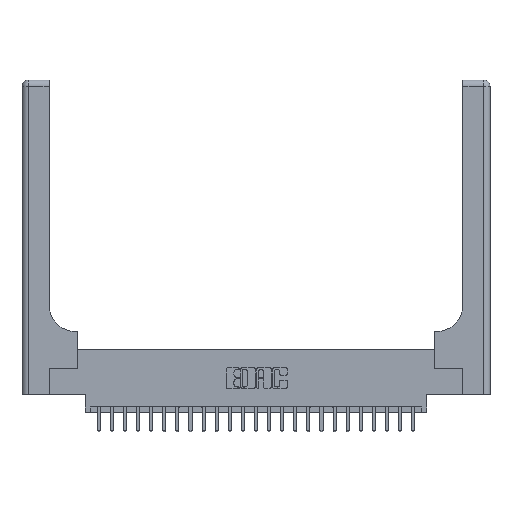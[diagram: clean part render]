
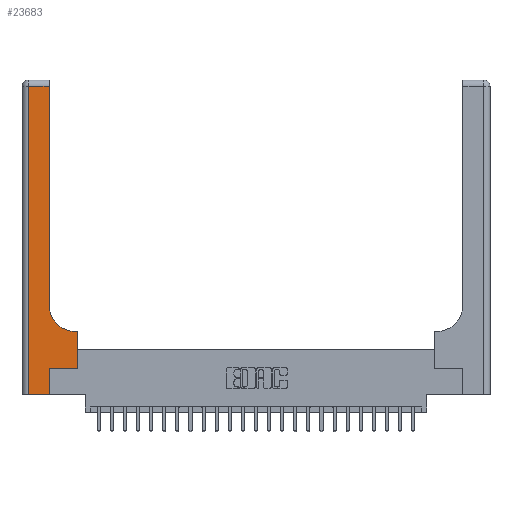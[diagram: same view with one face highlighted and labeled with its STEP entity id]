
A CAD part, top view. The second image highlights one B-rep face of the part: STEP entity #23683.
In plain terms, the highlighted planar face has unit normal (0, 0, 1).
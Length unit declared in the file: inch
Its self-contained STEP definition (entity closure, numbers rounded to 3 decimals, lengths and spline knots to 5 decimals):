
#75 = LINE ( 'NONE', #4916, #19476 ) ;
#496 = VECTOR ( 'NONE', #17481, 39.37008 ) ;
#498 = VERTEX_POINT ( 'NONE', #15207 ) ;
#899 = VECTOR ( 'NONE', #15402, 39.37008 ) ;
#1504 = EDGE_CURVE ( 'NONE', #498, #10730, #18306, .T. ) ;
#1508 = LINE ( 'NONE', #15621, #899 ) ;
#1638 = EDGE_CURVE ( 'NONE', #2886, #498, #1508, .T. ) ;
#1781 = CARTESIAN_POINT ( 'NONE',  ( 0., 0., 0.37 ) ) ;
#1976 = EDGE_CURVE ( 'NONE', #14394, #15338, #6405, .T. ) ;
#2412 = ORIENTED_EDGE ( 'NONE', *, *, #1504, .T. ) ;
#2886 = VERTEX_POINT ( 'NONE', #19608 ) ;
#3238 = CIRCLE ( 'NONE', #21784, 0.25 ) ;
#3376 = VECTOR ( 'NONE', #17264, 39.37008 ) ;
#3769 = DIRECTION ( 'NONE',  ( 1., 0., 0. ) ) ;
#4017 = VECTOR ( 'NONE', #19359, 39.37008 ) ;
#4761 = EDGE_CURVE ( 'NONE', #8968, #14394, #22690, .T. ) ;
#4916 = CARTESIAN_POINT ( 'NONE',  ( 0.528, 0.25, 0.37 ) ) ;
#4970 = DIRECTION ( 'NONE',  ( -1., 0., 0. ) ) ;
#5812 = VERTEX_POINT ( 'NONE', #20276 ) ;
#6086 = FACE_OUTER_BOUND ( 'NONE', #12149, .T. ) ;
#6405 = LINE ( 'NONE', #12341, #14629 ) ;
#6441 = ORIENTED_EDGE ( 'NONE', *, *, #17132, .T. ) ;
#6444 = CARTESIAN_POINT ( 'NONE',  ( 0.06, 3., 0.37 ) ) ;
#6868 = ORIENTED_EDGE ( 'NONE', *, *, #20390, .T. ) ;
#6912 = CARTESIAN_POINT ( 'NONE',  ( 0.528, 0.6, 0.37 ) ) ;
#7313 = CARTESIAN_POINT ( 'NONE',  ( 0.528, 0.25, 0.37 ) ) ;
#7423 = EDGE_CURVE ( 'NONE', #15338, #20185, #75, .T. ) ;
#7747 = DIRECTION ( 'NONE',  ( 0., 0., -1. ) ) ;
#8833 = ORIENTED_EDGE ( 'NONE', *, *, #19683, .T. ) ;
#8968 = VERTEX_POINT ( 'NONE', #13856 ) ;
#10386 = ORIENTED_EDGE ( 'NONE', *, *, #7423, .T. ) ;
#10729 = ORIENTED_EDGE ( 'NONE', *, *, #1638, .T. ) ;
#10730 = VERTEX_POINT ( 'NONE', #11451 ) ;
#11451 = CARTESIAN_POINT ( 'NONE',  ( 0.06, 2.94, 0.37 ) ) ;
#12149 = EDGE_LOOP ( 'NONE', ( #10729, #2412, #22836, #6441, #19421, #19979, #10386, #8833, #6868 ) ) ;
#12291 = DIRECTION ( 'NONE',  ( 1., 0., 0. ) ) ;
#12341 = CARTESIAN_POINT ( 'NONE',  ( 0.265, 0.25, 0.37 ) ) ;
#12396 = LINE ( 'NONE', #1781, #21416 ) ;
#12555 = VECTOR ( 'NONE', #16365, 39.37008 ) ;
#12733 = EDGE_CURVE ( 'NONE', #10730, #23646, #18889, .T. ) ;
#13856 = CARTESIAN_POINT ( 'NONE',  ( 0.265, 0., 0.37 ) ) ;
#14313 = CARTESIAN_POINT ( 'NONE',  ( 0., 3., 0.37 ) ) ;
#14394 = VERTEX_POINT ( 'NONE', #22449 ) ;
#14417 = DIRECTION ( 'NONE',  ( 0., 1., 0. ) ) ;
#14629 = VECTOR ( 'NONE', #12291, 39.37008 ) ;
#15207 = CARTESIAN_POINT ( 'NONE',  ( 0.26, 2.94, 0.37 ) ) ;
#15338 = VERTEX_POINT ( 'NONE', #7313 ) ;
#15402 = DIRECTION ( 'NONE',  ( 0., 1., 0. ) ) ;
#15621 = CARTESIAN_POINT ( 'NONE',  ( 0.26, 3., 0.37 ) ) ;
#16179 = DIRECTION ( 'NONE',  ( 0., 0., -1. ) ) ;
#16365 = DIRECTION ( 'NONE',  ( -1., 0., 0. ) ) ;
#17132 = EDGE_CURVE ( 'NONE', #23646, #8968, #12396, .T. ) ;
#17264 = DIRECTION ( 'NONE',  ( -1., 0., 0. ) ) ;
#17306 = AXIS2_PLACEMENT_3D ( 'NONE', #14313, #16179, #4970 ) ;
#17481 = DIRECTION ( 'NONE',  ( 0., 1., 0. ) ) ;
#17650 = CARTESIAN_POINT ( 'NONE',  ( 0., 2.94, 0.37 ) ) ;
#18306 = LINE ( 'NONE', #17650, #3376 ) ;
#18787 = CARTESIAN_POINT ( 'NONE',  ( 0.51, 0.85, 0.37 ) ) ;
#18889 = LINE ( 'NONE', #6444, #4017 ) ;
#19292 = CARTESIAN_POINT ( 'NONE',  ( 0.265, 0., 0.37 ) ) ;
#19359 = DIRECTION ( 'NONE',  ( 0., -1., 0. ) ) ;
#19421 = ORIENTED_EDGE ( 'NONE', *, *, #4761, .T. ) ;
#19476 = VECTOR ( 'NONE', #14417, 39.37008 ) ;
#19608 = CARTESIAN_POINT ( 'NONE',  ( 0.26, 0.85, 0.37 ) ) ;
#19683 = EDGE_CURVE ( 'NONE', #20185, #5812, #22145, .T. ) ;
#19737 = PLANE ( 'NONE',  #17306 ) ;
#19979 = ORIENTED_EDGE ( 'NONE', *, *, #1976, .T. ) ;
#20185 = VERTEX_POINT ( 'NONE', #6912 ) ;
#20276 = CARTESIAN_POINT ( 'NONE',  ( 0.51, 0.6, 0.37 ) ) ;
#20390 = EDGE_CURVE ( 'NONE', #5812, #2886, #3238, .T. ) ;
#20593 = DIRECTION ( 'NONE',  ( 1., 0., 0. ) ) ;
#21416 = VECTOR ( 'NONE', #3769, 39.37008 ) ;
#21711 = CARTESIAN_POINT ( 'NONE',  ( 0.26, 0.6, 0.37 ) ) ;
#21784 = AXIS2_PLACEMENT_3D ( 'NONE', #18787, #7747, #20593 ) ;
#22145 = LINE ( 'NONE', #21711, #12555 ) ;
#22449 = CARTESIAN_POINT ( 'NONE',  ( 0.265, 0.25, 0.37 ) ) ;
#22690 = LINE ( 'NONE', #19292, #496 ) ;
#22836 = ORIENTED_EDGE ( 'NONE', *, *, #12733, .T. ) ;
#23242 = CARTESIAN_POINT ( 'NONE',  ( 0.06, 0., 0.37 ) ) ;
#23646 = VERTEX_POINT ( 'NONE', #23242 ) ;
#23683 = ADVANCED_FACE ( 'NONE', ( #6086 ), #19737, .F. ) ;
